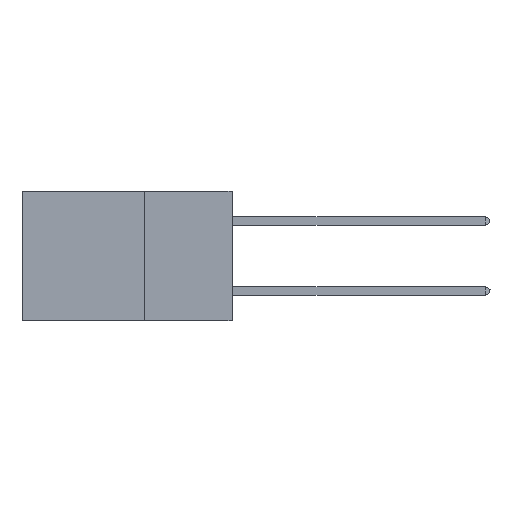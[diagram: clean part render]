
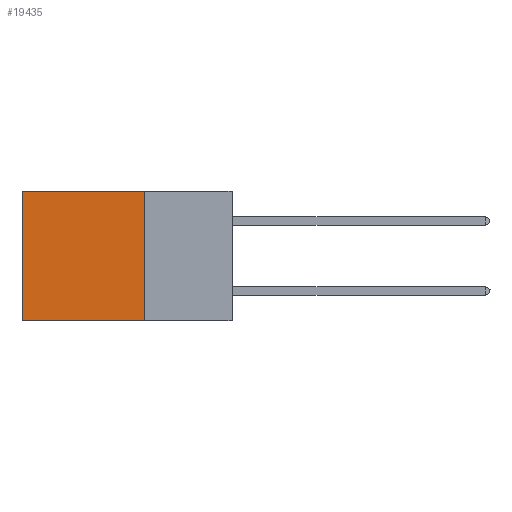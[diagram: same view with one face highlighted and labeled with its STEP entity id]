
A CAD part, left-side view. The second image highlights one B-rep face of the part: STEP entity #19435.
In plain terms, the highlighted planar face has unit normal (-1, 0, 0).
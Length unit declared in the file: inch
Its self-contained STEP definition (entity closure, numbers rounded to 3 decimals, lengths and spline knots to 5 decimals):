
#2521 = CARTESIAN_POINT ( 'NONE',  ( 0.2875, 0.25, 0. ) ) ;
#2706 = VECTOR ( 'NONE', #22540, 39.37008 ) ;
#3329 = VERTEX_POINT ( 'NONE', #23103 ) ;
#4050 = ORIENTED_EDGE ( 'NONE', *, *, #7668, .T. ) ;
#6035 = LINE ( 'NONE', #25310, #22897 ) ;
#6041 = AXIS2_PLACEMENT_3D ( 'NONE', #20374, #20655, #13487 ) ;
#7231 = PLANE ( 'NONE',  #6041 ) ;
#7668 = EDGE_CURVE ( 'NONE', #23735, #24037, #21639, .T. ) ;
#8204 = CARTESIAN_POINT ( 'NONE',  ( 0.2875, 0.25, 0. ) ) ;
#8489 = CARTESIAN_POINT ( 'NONE',  ( 0.2875, 0.6, 0. ) ) ;
#9632 = DIRECTION ( 'NONE',  ( 0., 1., 0. ) ) ;
#11786 = LINE ( 'NONE', #22225, #19764 ) ;
#12260 = ORIENTED_EDGE ( 'NONE', *, *, #15520, .T. ) ;
#12372 = ORIENTED_EDGE ( 'NONE', *, *, #20189, .F. ) ;
#12480 = DIRECTION ( 'NONE',  ( 0., 0., -1. ) ) ;
#12946 = VERTEX_POINT ( 'NONE', #8204 ) ;
#13487 = DIRECTION ( 'NONE',  ( 0., 0., -1. ) ) ;
#13960 = VECTOR ( 'NONE', #12480, 39.37008 ) ;
#14454 = DIRECTION ( 'NONE',  ( 0., 0., -1. ) ) ;
#15520 = EDGE_CURVE ( 'NONE', #12946, #23735, #22684, .T. ) ;
#18486 = FACE_OUTER_BOUND ( 'NONE', #24275, .T. ) ;
#19435 = ADVANCED_FACE ( 'NONE', ( #18486 ), #7231, .F. ) ;
#19764 = VECTOR ( 'NONE', #9632, 39.37008 ) ;
#20189 = EDGE_CURVE ( 'NONE', #3329, #24037, #11786, .T. ) ;
#20374 = CARTESIAN_POINT ( 'NONE',  ( 0.2875, 0.25, 0. ) ) ;
#20655 = DIRECTION ( 'NONE',  ( 1., 0., 0. ) ) ;
#21639 = LINE ( 'NONE', #8489, #13960 ) ;
#22225 = CARTESIAN_POINT ( 'NONE',  ( 0.2875, 0.25, -0.37 ) ) ;
#22540 = DIRECTION ( 'NONE',  ( 0., 1., 0. ) ) ;
#22684 = LINE ( 'NONE', #2521, #2706 ) ;
#22897 = VECTOR ( 'NONE', #14454, 39.37008 ) ;
#23103 = CARTESIAN_POINT ( 'NONE',  ( 0.2875, 0.25, -0.37 ) ) ;
#23295 = CARTESIAN_POINT ( 'NONE',  ( 0.2875, 0.6, -0.37 ) ) ;
#23497 = EDGE_CURVE ( 'NONE', #12946, #3329, #6035, .T. ) ;
#23735 = VERTEX_POINT ( 'NONE', #24154 ) ;
#24037 = VERTEX_POINT ( 'NONE', #23295 ) ;
#24154 = CARTESIAN_POINT ( 'NONE',  ( 0.2875, 0.6, 0. ) ) ;
#24275 = EDGE_LOOP ( 'NONE', ( #4050, #12372, #26226, #12260 ) ) ;
#25310 = CARTESIAN_POINT ( 'NONE',  ( 0.2875, 0.25, 0. ) ) ;
#26226 = ORIENTED_EDGE ( 'NONE', *, *, #23497, .F. ) ;
